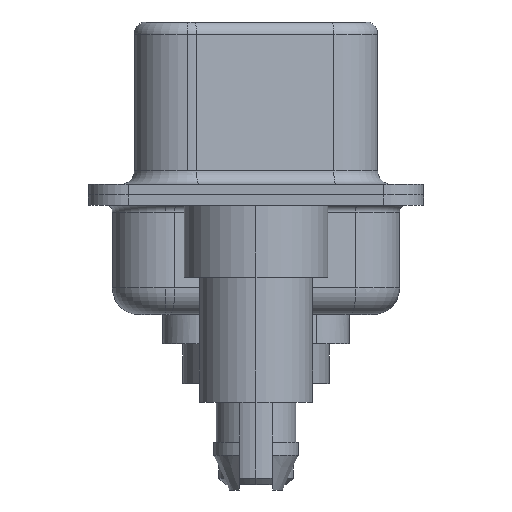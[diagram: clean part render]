
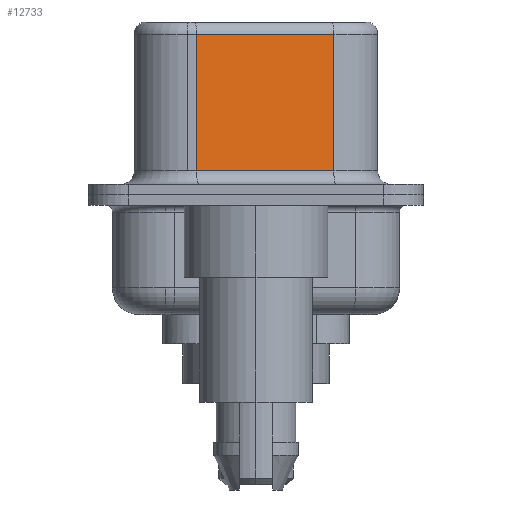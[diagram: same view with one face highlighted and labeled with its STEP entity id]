
A CAD part, left-side view. The second image highlights one B-rep face of the part: STEP entity #12733.
In plain terms, the highlighted planar face has unit normal (-0.985, -0.174, 0).
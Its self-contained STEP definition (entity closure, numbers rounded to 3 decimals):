
#149 = DIRECTION ( 'NONE',  ( 0.174, -0.985, 0. ) ) ;
#263 = AXIS2_PLACEMENT_3D ( 'NONE', #3941, #6306, #14472 ) ;
#897 = EDGE_LOOP ( 'NONE', ( #5561, #11015, #12306, #5235 ) ) ;
#1300 = CARTESIAN_POINT ( 'NONE',  ( 4.58, -2.927, 6.02 ) ) ;
#1697 = VERTEX_POINT ( 'NONE', #3985 ) ;
#1965 = CARTESIAN_POINT ( 'NONE',  ( 4.58, -2.927, 6.02 ) ) ;
#2399 = EDGE_CURVE ( 'NONE', #13999, #7281, #12962, .T. ) ;
#2658 = DIRECTION ( 'NONE',  ( 0., 0., -1. ) ) ;
#2700 = FACE_OUTER_BOUND ( 'NONE', #897, .T. ) ;
#3941 = CARTESIAN_POINT ( 'NONE',  ( 4.58, -2.927, 6.52 ) ) ;
#3985 = CARTESIAN_POINT ( 'NONE',  ( 3.67, 2.233, 6.02 ) ) ;
#4753 = EDGE_CURVE ( 'NONE', #14064, #7281, #13629, .T. ) ;
#5235 = ORIENTED_EDGE ( 'NONE', *, *, #2399, .T. ) ;
#5359 = CARTESIAN_POINT ( 'NONE',  ( 3.67, 2.233, 0.9 ) ) ;
#5480 = VECTOR ( 'NONE', #2658, 1000. ) ;
#5561 = ORIENTED_EDGE ( 'NONE', *, *, #4753, .F. ) ;
#5804 = VECTOR ( 'NONE', #13022, 1000. ) ;
#6306 = DIRECTION ( 'NONE',  ( 0.985, 0.174, 0. ) ) ;
#7281 = VERTEX_POINT ( 'NONE', #11446 ) ;
#8973 = LINE ( 'NONE', #10887, #5480 ) ;
#9699 = DIRECTION ( 'NONE',  ( 0., 0., -1. ) ) ;
#9870 = VECTOR ( 'NONE', #149, 1000. ) ;
#10501 = CARTESIAN_POINT ( 'NONE',  ( 4.58, -2.927, 0.9 ) ) ;
#10565 = VECTOR ( 'NONE', #9699, 1000. ) ;
#10887 = CARTESIAN_POINT ( 'NONE',  ( 3.67, 2.233, 6.52 ) ) ;
#11015 = ORIENTED_EDGE ( 'NONE', *, *, #13846, .T. ) ;
#11446 = CARTESIAN_POINT ( 'NONE',  ( 4.58, -2.927, 0.9 ) ) ;
#11552 = EDGE_CURVE ( 'NONE', #1697, #13999, #8973, .T. ) ;
#12100 = CARTESIAN_POINT ( 'NONE',  ( 4.58, -2.927, 6.52 ) ) ;
#12124 = PLANE ( 'NONE',  #263 ) ;
#12306 = ORIENTED_EDGE ( 'NONE', *, *, #11552, .T. ) ;
#12401 = LINE ( 'NONE', #1300, #5804 ) ;
#12733 = ADVANCED_FACE ( 'NONE', ( #2700 ), #12124, .F. ) ;
#12962 = LINE ( 'NONE', #10501, #9870 ) ;
#13022 = DIRECTION ( 'NONE',  ( -0.174, 0.985, 0. ) ) ;
#13629 = LINE ( 'NONE', #12100, #10565 ) ;
#13846 = EDGE_CURVE ( 'NONE', #14064, #1697, #12401, .T. ) ;
#13999 = VERTEX_POINT ( 'NONE', #5359 ) ;
#14064 = VERTEX_POINT ( 'NONE', #1965 ) ;
#14472 = DIRECTION ( 'NONE',  ( -0.174, 0.985, 0. ) ) ;
